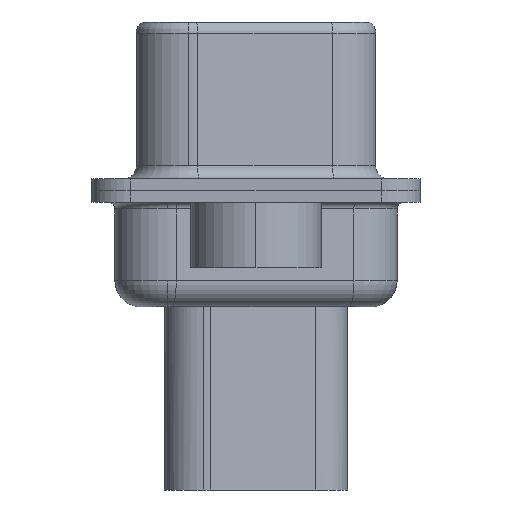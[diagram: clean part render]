
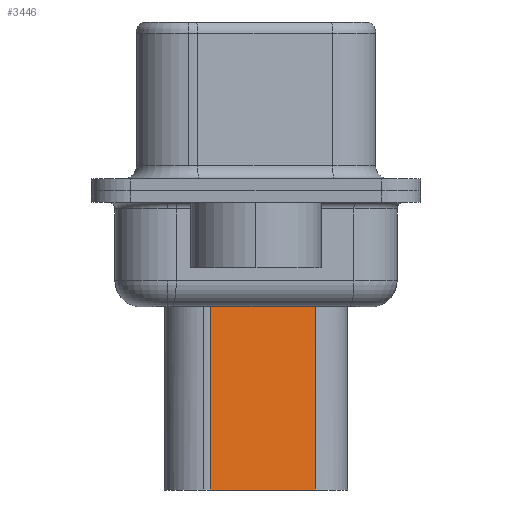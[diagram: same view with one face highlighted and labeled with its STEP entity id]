
A CAD part, left-side view. The second image highlights one B-rep face of the part: STEP entity #3446.
In plain terms, the highlighted planar face has unit normal (-0.985, -0.174, 0).
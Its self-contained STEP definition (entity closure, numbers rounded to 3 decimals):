
#550 = EDGE_CURVE ( 'NONE', #1469, #17391, #15734, .T. ) ;
#849 = VECTOR ( 'NONE', #7332, 1000. ) ;
#1080 = EDGE_CURVE ( 'NONE', #7343, #2879, #6812, .T. ) ;
#1469 = VERTEX_POINT ( 'NONE', #17044 ) ;
#1628 = LINE ( 'NONE', #3756, #16086 ) ;
#2874 = PLANE ( 'NONE',  #14409 ) ;
#2879 = VERTEX_POINT ( 'NONE', #8675 ) ;
#3087 = VECTOR ( 'NONE', #4480, 1000. ) ;
#3446 = ADVANCED_FACE ( 'NONE', ( #5003 ), #2874, .T. ) ;
#3756 = CARTESIAN_POINT ( 'NONE',  ( 4.353, 2.709, -3.975 ) ) ;
#4035 = ORIENTED_EDGE ( 'NONE', *, *, #12210, .F. ) ;
#4197 = ORIENTED_EDGE ( 'NONE', *, *, #550, .T. ) ;
#4243 = CARTESIAN_POINT ( 'NONE',  ( 5.229, -2.26, -3.1 ) ) ;
#4480 = DIRECTION ( 'NONE',  ( 0., 0., -1. ) ) ;
#4674 = ORIENTED_EDGE ( 'NONE', *, *, #1080, .F. ) ;
#5003 = FACE_OUTER_BOUND ( 'NONE', #14309, .T. ) ;
#5178 = EDGE_CURVE ( 'NONE', #7343, #1469, #1628, .T. ) ;
#6201 = DIRECTION ( 'NONE',  ( -0.174, 0.985, 0. ) ) ;
#6476 = LINE ( 'NONE', #10424, #13494 ) ;
#6812 = LINE ( 'NONE', #4243, #3087 ) ;
#7332 = DIRECTION ( 'NONE',  ( 0., 0., -1. ) ) ;
#7343 = VERTEX_POINT ( 'NONE', #17676 ) ;
#8675 = CARTESIAN_POINT ( 'NONE',  ( 5.229, -2.26, -11.45 ) ) ;
#9374 = DIRECTION ( 'NONE',  ( -0.174, 0.985, 0. ) ) ;
#10424 = CARTESIAN_POINT ( 'NONE',  ( 4.524, 1.74, -11.45 ) ) ;
#12210 = EDGE_CURVE ( 'NONE', #2879, #17391, #6476, .T. ) ;
#13494 = VECTOR ( 'NONE', #6201, 1000. ) ;
#14309 = EDGE_LOOP ( 'NONE', ( #4674, #14724, #4197, #4035 ) ) ;
#14409 = AXIS2_PLACEMENT_3D ( 'NONE', #16727, #16024, #15962 ) ;
#14621 = CARTESIAN_POINT ( 'NONE',  ( 4.524, 1.74, -11.45 ) ) ;
#14724 = ORIENTED_EDGE ( 'NONE', *, *, #5178, .T. ) ;
#15727 = CARTESIAN_POINT ( 'NONE',  ( 4.524, 1.74, -3.1 ) ) ;
#15734 = LINE ( 'NONE', #15727, #849 ) ;
#15962 = DIRECTION ( 'NONE',  ( 0.174, -0.985, 0. ) ) ;
#16024 = DIRECTION ( 'NONE',  ( -0.985, -0.174, 0. ) ) ;
#16086 = VECTOR ( 'NONE', #9374, 1000. ) ;
#16727 = CARTESIAN_POINT ( 'NONE',  ( 4.524, 1.74, -3.1 ) ) ;
#17044 = CARTESIAN_POINT ( 'NONE',  ( 4.524, 1.74, -3.975 ) ) ;
#17391 = VERTEX_POINT ( 'NONE', #14621 ) ;
#17676 = CARTESIAN_POINT ( 'NONE',  ( 5.229, -2.26, -3.975 ) ) ;
